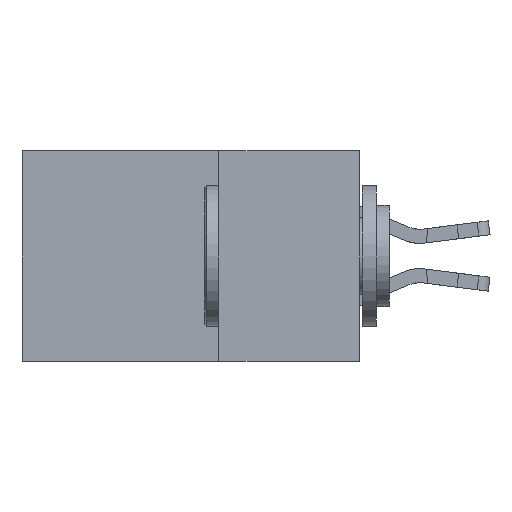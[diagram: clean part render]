
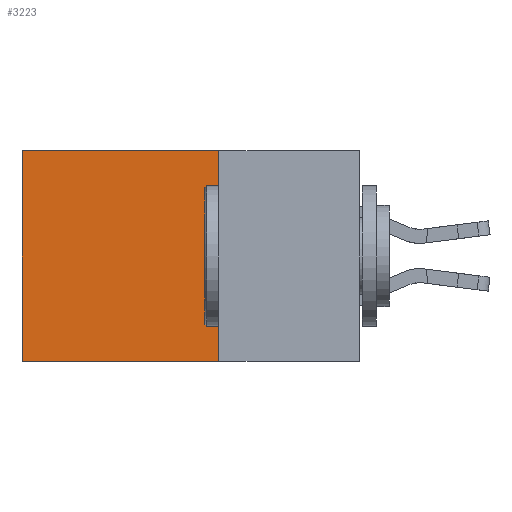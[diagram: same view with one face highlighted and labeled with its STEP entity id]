
A CAD part, left-side view. The second image highlights one B-rep face of the part: STEP entity #3223.
In plain terms, the highlighted planar face has unit normal (-1, 0, 0).
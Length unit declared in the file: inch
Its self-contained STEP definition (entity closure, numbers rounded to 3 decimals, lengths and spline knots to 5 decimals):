
#34 = EDGE_LOOP ( 'NONE', ( #16594, #8603, #4369, #15040 ) ) ;
#932 = CARTESIAN_POINT ( 'NONE',  ( 0.2875, 0.25, -0.375 ) ) ;
#1831 = DIRECTION ( 'NONE',  ( 0., 0., -1. ) ) ;
#2815 = DIRECTION ( 'NONE',  ( 1., 0., 0. ) ) ;
#2893 = EDGE_CURVE ( 'NONE', #9890, #18538, #18758, .T. ) ;
#3177 = FACE_OUTER_BOUND ( 'NONE', #34, .T. ) ;
#3223 = ADVANCED_FACE ( 'NONE', ( #3177 ), #16658, .F. ) ;
#3631 = EDGE_CURVE ( 'NONE', #6736, #18538, #17750, .T. ) ;
#4346 = CARTESIAN_POINT ( 'NONE',  ( 0.2875, 0.25, -0.375 ) ) ;
#4369 = ORIENTED_EDGE ( 'NONE', *, *, #19467, .F. ) ;
#4904 = LINE ( 'NONE', #12213, #18302 ) ;
#6581 = EDGE_CURVE ( 'NONE', #8816, #9890, #4904, .T. ) ;
#6736 = VERTEX_POINT ( 'NONE', #19237 ) ;
#8603 = ORIENTED_EDGE ( 'NONE', *, *, #3631, .F. ) ;
#8816 = VERTEX_POINT ( 'NONE', #13740 ) ;
#9659 = VECTOR ( 'NONE', #1831, 39.37008 ) ;
#9890 = VERTEX_POINT ( 'NONE', #12745 ) ;
#10622 = DIRECTION ( 'NONE',  ( 0., 1., 0. ) ) ;
#10997 = DIRECTION ( 'NONE',  ( 0., 0., -1. ) ) ;
#12103 = AXIS2_PLACEMENT_3D ( 'NONE', #4346, #2815, #16597 ) ;
#12213 = CARTESIAN_POINT ( 'NONE',  ( 0.2875, 0.25, 0. ) ) ;
#12467 = LINE ( 'NONE', #15589, #12708 ) ;
#12708 = VECTOR ( 'NONE', #10997, 39.37008 ) ;
#12745 = CARTESIAN_POINT ( 'NONE',  ( 0.2875, 0.6, 0. ) ) ;
#13220 = CARTESIAN_POINT ( 'NONE',  ( 0.2875, 0.6, -0.375 ) ) ;
#13228 = DIRECTION ( 'NONE',  ( 0., 1., 0. ) ) ;
#13740 = CARTESIAN_POINT ( 'NONE',  ( 0.2875, 0.25, 0. ) ) ;
#15040 = ORIENTED_EDGE ( 'NONE', *, *, #6581, .T. ) ;
#15589 = CARTESIAN_POINT ( 'NONE',  ( 0.2875, 0.25, -0.375 ) ) ;
#16594 = ORIENTED_EDGE ( 'NONE', *, *, #2893, .T. ) ;
#16597 = DIRECTION ( 'NONE',  ( 0., 0., -1. ) ) ;
#16658 = PLANE ( 'NONE',  #12103 ) ;
#17071 = CARTESIAN_POINT ( 'NONE',  ( 0.2875, 0.6, -0.375 ) ) ;
#17287 = VECTOR ( 'NONE', #13228, 39.37008 ) ;
#17750 = LINE ( 'NONE', #932, #17287 ) ;
#18302 = VECTOR ( 'NONE', #10622, 39.37008 ) ;
#18538 = VERTEX_POINT ( 'NONE', #13220 ) ;
#18758 = LINE ( 'NONE', #17071, #9659 ) ;
#19237 = CARTESIAN_POINT ( 'NONE',  ( 0.2875, 0.25, -0.375 ) ) ;
#19467 = EDGE_CURVE ( 'NONE', #8816, #6736, #12467, .T. ) ;
